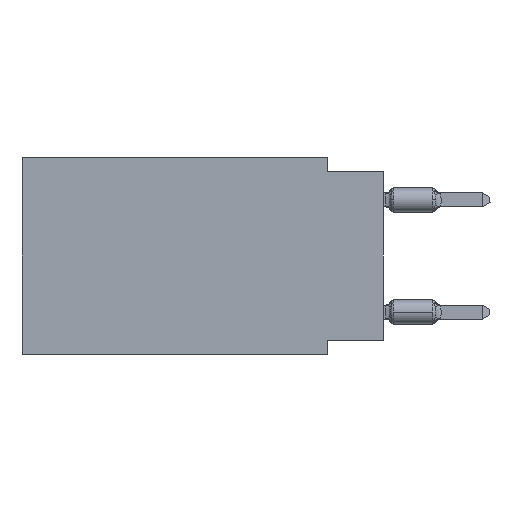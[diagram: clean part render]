
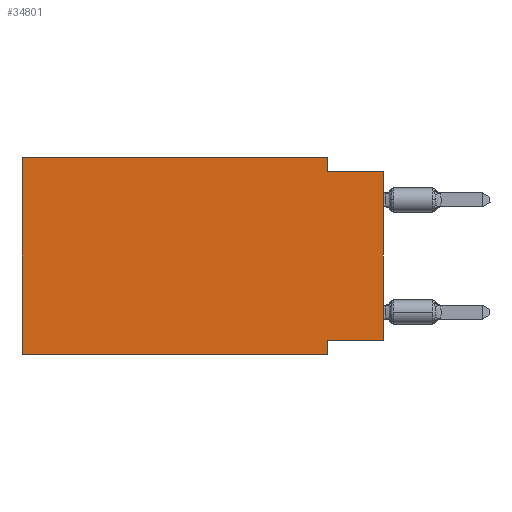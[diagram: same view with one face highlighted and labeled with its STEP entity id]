
A CAD part, left-side view. The second image highlights one B-rep face of the part: STEP entity #34801.
In plain terms, the highlighted planar face has unit normal (-1, 0, 0).
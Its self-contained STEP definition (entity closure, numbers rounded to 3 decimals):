
#999 = EDGE_CURVE ( 'NONE', #18801, #33451, #30674, .T. ) ;
#1134 = VECTOR ( 'NONE', #22771, 1000. ) ;
#1818 = DIRECTION ( 'NONE',  ( 0., 0., 1. ) ) ;
#2176 = VERTEX_POINT ( 'NONE', #25158 ) ;
#2639 = CARTESIAN_POINT ( 'NONE',  ( 0., 2.54, -8.89 ) ) ;
#3535 = VECTOR ( 'NONE', #20605, 1000. ) ;
#3844 = EDGE_CURVE ( 'NONE', #5880, #2176, #30946, .T. ) ;
#4265 = CARTESIAN_POINT ( 'NONE',  ( 0., 16.383, 0. ) ) ;
#5200 = ORIENTED_EDGE ( 'NONE', *, *, #23012, .F. ) ;
#5518 = DIRECTION ( 'NONE',  ( 0., -1., 0. ) ) ;
#5774 = EDGE_CURVE ( 'NONE', #22762, #33451, #39500, .T. ) ;
#5880 = VERTEX_POINT ( 'NONE', #25523 ) ;
#6613 = CARTESIAN_POINT ( 'NONE',  ( 0., 2.54, 0. ) ) ;
#6930 = CARTESIAN_POINT ( 'NONE',  ( 0., 2.54, -0.635 ) ) ;
#7321 = LINE ( 'NONE', #26137, #3535 ) ;
#7704 = DIRECTION ( 'NONE',  ( 0., 1., 0. ) ) ;
#8376 = CARTESIAN_POINT ( 'NONE',  ( 0., 16.383, -8.89 ) ) ;
#8695 = EDGE_LOOP ( 'NONE', ( #31788, #17807, #5200, #16120, #26513, #29225, #16279, #19386 ) ) ;
#10718 = DIRECTION ( 'NONE',  ( 1., 0., 0. ) ) ;
#11124 = PLANE ( 'NONE',  #14143 ) ;
#13827 = LINE ( 'NONE', #26300, #37908 ) ;
#14143 = AXIS2_PLACEMENT_3D ( 'NONE', #35687, #10718, #14195 ) ;
#14169 = LINE ( 'NONE', #35446, #39022 ) ;
#14195 = DIRECTION ( 'NONE',  ( 0., 0., -1. ) ) ;
#14796 = CARTESIAN_POINT ( 'NONE',  ( 0., 0., 0. ) ) ;
#16120 = ORIENTED_EDGE ( 'NONE', *, *, #20298, .F. ) ;
#16279 = ORIENTED_EDGE ( 'NONE', *, *, #5774, .F. ) ;
#17807 = ORIENTED_EDGE ( 'NONE', *, *, #19636, .F. ) ;
#17946 = LINE ( 'NONE', #39268, #28264 ) ;
#18018 = VERTEX_POINT ( 'NONE', #4265 ) ;
#18801 = VERTEX_POINT ( 'NONE', #35398 ) ;
#19386 = ORIENTED_EDGE ( 'NONE', *, *, #39980, .F. ) ;
#19572 = VERTEX_POINT ( 'NONE', #6613 ) ;
#19636 = EDGE_CURVE ( 'NONE', #25313, #2176, #14169, .T. ) ;
#20298 = EDGE_CURVE ( 'NONE', #18018, #19572, #35084, .T. ) ;
#20605 = DIRECTION ( 'NONE',  ( 0., 0., -1. ) ) ;
#21526 = VECTOR ( 'NONE', #5518, 1000. ) ;
#22733 = VECTOR ( 'NONE', #30469, 1000. ) ;
#22762 = VERTEX_POINT ( 'NONE', #24528 ) ;
#22771 = DIRECTION ( 'NONE',  ( 0., -1., 0. ) ) ;
#23012 = EDGE_CURVE ( 'NONE', #19572, #25313, #7321, .T. ) ;
#24528 = CARTESIAN_POINT ( 'NONE',  ( 0., 2.54, -8.255 ) ) ;
#24597 = DIRECTION ( 'NONE',  ( 0., 0., 1. ) ) ;
#25158 = CARTESIAN_POINT ( 'NONE',  ( 0., 0., -0.635 ) ) ;
#25313 = VERTEX_POINT ( 'NONE', #6930 ) ;
#25523 = CARTESIAN_POINT ( 'NONE',  ( 0., 0., -8.255 ) ) ;
#26137 = CARTESIAN_POINT ( 'NONE',  ( 0., 2.54, 0. ) ) ;
#26300 = CARTESIAN_POINT ( 'NONE',  ( 0., 0., -8.255 ) ) ;
#26467 = FACE_OUTER_BOUND ( 'NONE', #8695, .T. ) ;
#26513 = ORIENTED_EDGE ( 'NONE', *, *, #31496, .F. ) ;
#28264 = VECTOR ( 'NONE', #1818, 1000. ) ;
#29225 = ORIENTED_EDGE ( 'NONE', *, *, #999, .T. ) ;
#30469 = DIRECTION ( 'NONE',  ( 0., 0., -1. ) ) ;
#30508 = VECTOR ( 'NONE', #24597, 1000. ) ;
#30674 = LINE ( 'NONE', #8376, #21526 ) ;
#30946 = LINE ( 'NONE', #14796, #30508 ) ;
#31496 = EDGE_CURVE ( 'NONE', #18801, #18018, #17946, .T. ) ;
#31788 = ORIENTED_EDGE ( 'NONE', *, *, #3844, .T. ) ;
#32623 = CARTESIAN_POINT ( 'NONE',  ( 0., 16.383, 0. ) ) ;
#32791 = DIRECTION ( 'NONE',  ( 0., -1., 0. ) ) ;
#33451 = VERTEX_POINT ( 'NONE', #39179 ) ;
#34801 = ADVANCED_FACE ( 'NONE', ( #26467 ), #11124, .F. ) ;
#35084 = LINE ( 'NONE', #32623, #1134 ) ;
#35398 = CARTESIAN_POINT ( 'NONE',  ( 0., 16.383, -8.89 ) ) ;
#35446 = CARTESIAN_POINT ( 'NONE',  ( 0., 0., -0.635 ) ) ;
#35687 = CARTESIAN_POINT ( 'NONE',  ( 0., 16.383, 0. ) ) ;
#37908 = VECTOR ( 'NONE', #7704, 1000. ) ;
#39022 = VECTOR ( 'NONE', #32791, 1000. ) ;
#39179 = CARTESIAN_POINT ( 'NONE',  ( 0., 2.54, -8.89 ) ) ;
#39268 = CARTESIAN_POINT ( 'NONE',  ( 0., 16.383, 0. ) ) ;
#39500 = LINE ( 'NONE', #2639, #22733 ) ;
#39980 = EDGE_CURVE ( 'NONE', #5880, #22762, #13827, .T. ) ;
